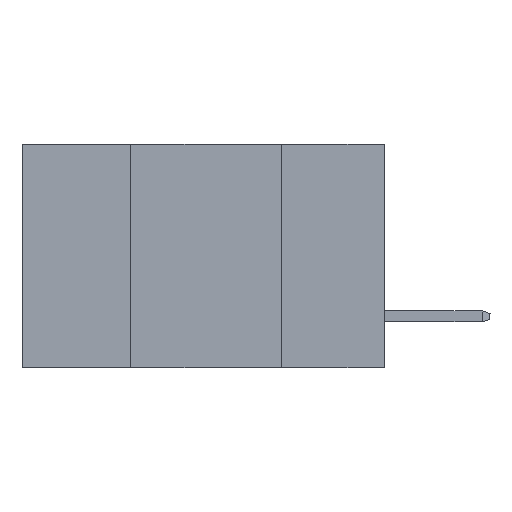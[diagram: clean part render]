
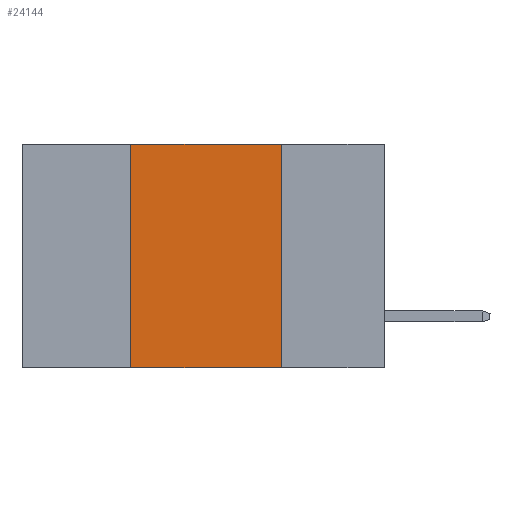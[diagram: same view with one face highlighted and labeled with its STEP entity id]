
A CAD part, left-side view. The second image highlights one B-rep face of the part: STEP entity #24144.
In plain terms, the highlighted planar face has unit normal (-1, 0, 0).
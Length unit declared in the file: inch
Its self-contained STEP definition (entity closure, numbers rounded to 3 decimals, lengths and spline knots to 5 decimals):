
#796 = CARTESIAN_POINT ( 'NONE',  ( 0., 0.42, 0. ) ) ;
#819 = LINE ( 'NONE', #14545, #8990 ) ;
#1497 = VECTOR ( 'NONE', #14350, 39.37008 ) ;
#1672 = ORIENTED_EDGE ( 'NONE', *, *, #14839, .F. ) ;
#2186 = EDGE_CURVE ( 'NONE', #3448, #6963, #15004, .T. ) ;
#3044 = EDGE_LOOP ( 'NONE', ( #16519, #5592, #1672, #4524 ) ) ;
#3292 = CARTESIAN_POINT ( 'NONE',  ( 0., 0.6, -0.37 ) ) ;
#3448 = VERTEX_POINT ( 'NONE', #10603 ) ;
#4524 = ORIENTED_EDGE ( 'NONE', *, *, #2186, .T. ) ;
#4607 = DIRECTION ( 'NONE',  ( 0., 0., 1. ) ) ;
#5043 = LINE ( 'NONE', #9700, #16235 ) ;
#5592 = ORIENTED_EDGE ( 'NONE', *, *, #13722, .F. ) ;
#6963 = VERTEX_POINT ( 'NONE', #19205 ) ;
#7191 = VERTEX_POINT ( 'NONE', #21663 ) ;
#8990 = VECTOR ( 'NONE', #4607, 39.37008 ) ;
#9700 = CARTESIAN_POINT ( 'NONE',  ( 0., 0.17, 0. ) ) ;
#10001 = EDGE_CURVE ( 'NONE', #7191, #6963, #5043, .T. ) ;
#10603 = CARTESIAN_POINT ( 'NONE',  ( 0., 0.42, -0.37 ) ) ;
#11319 = DIRECTION ( 'NONE',  ( 0., 0., -1. ) ) ;
#11708 = DIRECTION ( 'NONE',  ( 0., 0., -1. ) ) ;
#11916 = PLANE ( 'NONE',  #15785 ) ;
#12135 = LINE ( 'NONE', #24501, #1497 ) ;
#12596 = FACE_OUTER_BOUND ( 'NONE', #3044, .T. ) ;
#13722 = EDGE_CURVE ( 'NONE', #22725, #7191, #12135, .T. ) ;
#14350 = DIRECTION ( 'NONE',  ( 0., -1., 0. ) ) ;
#14545 = CARTESIAN_POINT ( 'NONE',  ( 0., 0.42, 0. ) ) ;
#14839 = EDGE_CURVE ( 'NONE', #3448, #22725, #819, .T. ) ;
#15004 = LINE ( 'NONE', #3292, #18127 ) ;
#15784 = CARTESIAN_POINT ( 'NONE',  ( 0., 0.6, 0. ) ) ;
#15785 = AXIS2_PLACEMENT_3D ( 'NONE', #15784, #15866, #11319 ) ;
#15866 = DIRECTION ( 'NONE',  ( 1., 0., 0. ) ) ;
#16235 = VECTOR ( 'NONE', #11708, 39.37008 ) ;
#16519 = ORIENTED_EDGE ( 'NONE', *, *, #10001, .F. ) ;
#18127 = VECTOR ( 'NONE', #25137, 39.37008 ) ;
#19205 = CARTESIAN_POINT ( 'NONE',  ( 0., 0.17, -0.37 ) ) ;
#21663 = CARTESIAN_POINT ( 'NONE',  ( 0., 0.17, 0. ) ) ;
#22725 = VERTEX_POINT ( 'NONE', #796 ) ;
#24144 = ADVANCED_FACE ( 'NONE', ( #12596 ), #11916, .F. ) ;
#24501 = CARTESIAN_POINT ( 'NONE',  ( 0., 0.6, 0. ) ) ;
#25137 = DIRECTION ( 'NONE',  ( 0., -1., 0. ) ) ;
